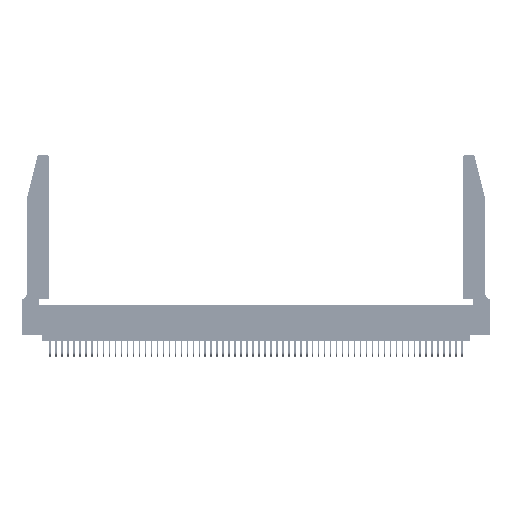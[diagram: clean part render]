
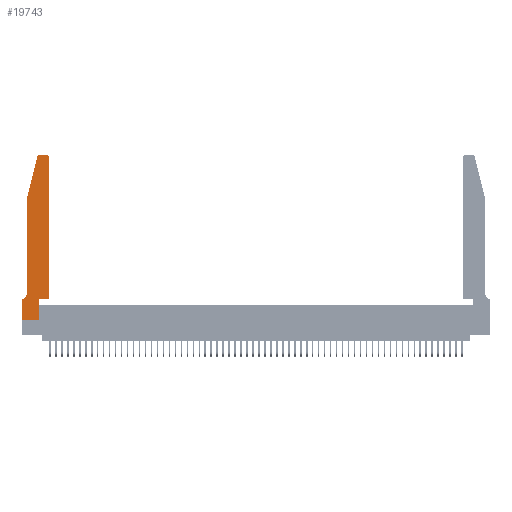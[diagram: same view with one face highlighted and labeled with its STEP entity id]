
A CAD part, top view. The second image highlights one B-rep face of the part: STEP entity #19743.
In plain terms, the highlighted planar face has unit normal (0, 0, 1).
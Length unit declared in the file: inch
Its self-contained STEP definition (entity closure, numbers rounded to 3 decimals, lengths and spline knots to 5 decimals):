
#25 = VERTEX_POINT ( 'NONE', #19618 ) ;
#184 = CARTESIAN_POINT ( 'NONE',  ( 0., 0., 0.37 ) ) ;
#414 = LINE ( 'NONE', #54785, #22951 ) ;
#1138 = PLANE ( 'NONE',  #3184 ) ;
#2138 = AXIS2_PLACEMENT_3D ( 'NONE', #4175, #35548, #8708 ) ;
#2216 = VECTOR ( 'NONE', #35121, 39.37008 ) ;
#3184 = AXIS2_PLACEMENT_3D ( 'NONE', #5700, #10213, #41513 ) ;
#3470 = CARTESIAN_POINT ( 'NONE',  ( 0., 0.35, 0.37 ) ) ;
#4175 = CARTESIAN_POINT ( 'NONE',  ( 0.4205, 2.72, 0.37 ) ) ;
#4857 = ORIENTED_EDGE ( 'NONE', *, *, #54850, .T. ) ;
#5116 = VECTOR ( 'NONE', #51935, 39.37008 ) ;
#5700 = CARTESIAN_POINT ( 'NONE',  ( 0., 0.35, 0.37 ) ) ;
#5824 = VECTOR ( 'NONE', #55251, 39.37008 ) ;
#6840 = EDGE_CURVE ( 'NONE', #33054, #10392, #52517, .T. ) ;
#7368 = EDGE_CURVE ( 'NONE', #10924, #45835, #23339, .T. ) ;
#8221 = CARTESIAN_POINT ( 'NONE',  ( 0.284, 2.75, 0.37 ) ) ;
#8708 = DIRECTION ( 'NONE',  ( 1., 0., 0. ) ) ;
#10213 = DIRECTION ( 'NONE',  ( 0., 0., 1. ) ) ;
#10296 = ORIENTED_EDGE ( 'NONE', *, *, #21707, .T. ) ;
#10392 = VERTEX_POINT ( 'NONE', #52893 ) ;
#10638 = EDGE_CURVE ( 'NONE', #51627, #43279, #414, .T. ) ;
#10670 = ORIENTED_EDGE ( 'NONE', *, *, #55352, .T. ) ;
#10924 = VERTEX_POINT ( 'NONE', #25758 ) ;
#13384 = VECTOR ( 'NONE', #36093, 39.37008 ) ;
#13732 = CARTESIAN_POINT ( 'NONE',  ( 0.2865, 0.35, 0.37 ) ) ;
#13821 = CARTESIAN_POINT ( 'NONE',  ( 0.0055, 0.42, 0.37 ) ) ;
#14497 = VERTEX_POINT ( 'NONE', #18834 ) ;
#14998 = EDGE_CURVE ( 'NONE', #38315, #31267, #20312, .T. ) ;
#16350 = CARTESIAN_POINT ( 'NONE',  ( 0., 0., 0.37 ) ) ;
#17699 = CARTESIAN_POINT ( 'NONE',  ( 0.4505, 0.35, 0.37 ) ) ;
#17760 = LINE ( 'NONE', #19375, #5824 ) ;
#18184 = ORIENTED_EDGE ( 'NONE', *, *, #10638, .T. ) ;
#18350 = DIRECTION ( 'NONE',  ( -1., 0., 0. ) ) ;
#18834 = CARTESIAN_POINT ( 'NONE',  ( 0.0755, 0.42, 0.37 ) ) ;
#19375 = CARTESIAN_POINT ( 'NONE',  ( 0.0755, 0.35, 0.37 ) ) ;
#19618 = CARTESIAN_POINT ( 'NONE',  ( 0.4505, 2.72, 0.37 ) ) ;
#19743 = ADVANCED_FACE ( 'NONE', ( #33979 ), #1138, .T. ) ;
#20312 = LINE ( 'NONE', #52967, #33606 ) ;
#20896 = ORIENTED_EDGE ( 'NONE', *, *, #50654, .T. ) ;
#21366 = DIRECTION ( 'NONE',  ( 0., 0., 1. ) ) ;
#21707 = EDGE_CURVE ( 'NONE', #10392, #10924, #48969, .T. ) ;
#22804 = CARTESIAN_POINT ( 'NONE',  ( 0.0755, 2., 0.37 ) ) ;
#22951 = VECTOR ( 'NONE', #50381, 39.37008 ) ;
#23339 = LINE ( 'NONE', #50955, #57281 ) ;
#23502 = DIRECTION ( 'NONE',  ( 1., 0., 0. ) ) ;
#24392 = DIRECTION ( 'NONE',  ( 0., 1., 0. ) ) ;
#25363 = LINE ( 'NONE', #27806, #47589 ) ;
#25570 = VERTEX_POINT ( 'NONE', #17699 ) ;
#25758 = CARTESIAN_POINT ( 'NONE',  ( 0.2865, 0., 0.37 ) ) ;
#26450 = DIRECTION ( 'NONE',  ( -0.239, -0.971, 0. ) ) ;
#27318 = DIRECTION ( 'NONE',  ( 0., -1., 0. ) ) ;
#27806 = CARTESIAN_POINT ( 'NONE',  ( 0.4505, 0.35, 0.37 ) ) ;
#28654 = VECTOR ( 'NONE', #27318, 39.37008 ) ;
#29739 = CIRCLE ( 'NONE', #55828, 0.03 ) ;
#30636 = CARTESIAN_POINT ( 'NONE',  ( 0.4505, 0.35, 0.37 ) ) ;
#31267 = VERTEX_POINT ( 'NONE', #38096 ) ;
#33031 = EDGE_CURVE ( 'NONE', #43279, #38315, #29739, .T. ) ;
#33054 = VERTEX_POINT ( 'NONE', #3470 ) ;
#33463 = EDGE_CURVE ( 'NONE', #35964, #33054, #17760, .T. ) ;
#33606 = VECTOR ( 'NONE', #26450, 39.37008 ) ;
#33979 = FACE_OUTER_BOUND ( 'NONE', #50938, .T. ) ;
#35121 = DIRECTION ( 'NONE',  ( 0., 1., 0. ) ) ;
#35139 = ORIENTED_EDGE ( 'NONE', *, *, #33031, .T. ) ;
#35548 = DIRECTION ( 'NONE',  ( 0., 0., 1. ) ) ;
#35964 = VERTEX_POINT ( 'NONE', #43340 ) ;
#36057 = AXIS2_PLACEMENT_3D ( 'NONE', #13821, #45080, #18350 ) ;
#36093 = DIRECTION ( 'NONE',  ( 1., 0., 0. ) ) ;
#38008 = LINE ( 'NONE', #30636, #2216 ) ;
#38096 = CARTESIAN_POINT ( 'NONE',  ( 0.0755, 2., 0.37 ) ) ;
#38315 = VERTEX_POINT ( 'NONE', #55022 ) ;
#39092 = ORIENTED_EDGE ( 'NONE', *, *, #51179, .T. ) ;
#40798 = EDGE_CURVE ( 'NONE', #31267, #14497, #47516, .T. ) ;
#41513 = DIRECTION ( 'NONE',  ( 1., 0., 0. ) ) ;
#42208 = CIRCLE ( 'NONE', #36057, 0.07 ) ;
#43279 = VERTEX_POINT ( 'NONE', #8221 ) ;
#43340 = CARTESIAN_POINT ( 'NONE',  ( 0.0055, 0.35, 0.37 ) ) ;
#44491 = ORIENTED_EDGE ( 'NONE', *, *, #7368, .T. ) ;
#44793 = CIRCLE ( 'NONE', #2138, 0.03 ) ;
#45080 = DIRECTION ( 'NONE',  ( 0., 0., -1. ) ) ;
#45835 = VERTEX_POINT ( 'NONE', #13732 ) ;
#46904 = ORIENTED_EDGE ( 'NONE', *, *, #40798, .T. ) ;
#47516 = LINE ( 'NONE', #22804, #28654 ) ;
#47589 = VECTOR ( 'NONE', #23502, 39.37008 ) ;
#48024 = CARTESIAN_POINT ( 'NONE',  ( 0.284, 2.72, 0.37 ) ) ;
#48461 = CARTESIAN_POINT ( 'NONE',  ( 0.4205, 2.75, 0.37 ) ) ;
#48969 = LINE ( 'NONE', #184, #13384 ) ;
#49507 = ORIENTED_EDGE ( 'NONE', *, *, #6840, .T. ) ;
#50381 = DIRECTION ( 'NONE',  ( -1., 0., 0. ) ) ;
#50654 = EDGE_CURVE ( 'NONE', #45835, #25570, #25363, .T. ) ;
#50938 = EDGE_LOOP ( 'NONE', ( #18184, #35139, #51770, #46904, #4857, #57687, #49507, #10296, #44491, #20896, #10670, #39092 ) ) ;
#50955 = CARTESIAN_POINT ( 'NONE',  ( 0.2865, 0.35, 0.37 ) ) ;
#51179 = EDGE_CURVE ( 'NONE', #25, #51627, #44793, .T. ) ;
#51627 = VERTEX_POINT ( 'NONE', #48461 ) ;
#51770 = ORIENTED_EDGE ( 'NONE', *, *, #14998, .T. ) ;
#51935 = DIRECTION ( 'NONE',  ( 0., -1., 0. ) ) ;
#52410 = DIRECTION ( 'NONE',  ( 1., 0., 0. ) ) ;
#52517 = LINE ( 'NONE', #16350, #5116 ) ;
#52893 = CARTESIAN_POINT ( 'NONE',  ( 0., 0., 0.37 ) ) ;
#52967 = CARTESIAN_POINT ( 'NONE',  ( 0.0755, 2., 0.37 ) ) ;
#54785 = CARTESIAN_POINT ( 'NONE',  ( 0.2605, 2.75, 0.37 ) ) ;
#54850 = EDGE_CURVE ( 'NONE', #14497, #35964, #42208, .T. ) ;
#55022 = CARTESIAN_POINT ( 'NONE',  ( 0.25487, 2.72718, 0.37 ) ) ;
#55251 = DIRECTION ( 'NONE',  ( -1., 0., 0. ) ) ;
#55352 = EDGE_CURVE ( 'NONE', #25570, #25, #38008, .T. ) ;
#55828 = AXIS2_PLACEMENT_3D ( 'NONE', #48024, #21366, #52410 ) ;
#57281 = VECTOR ( 'NONE', #24392, 39.37008 ) ;
#57687 = ORIENTED_EDGE ( 'NONE', *, *, #33463, .T. ) ;
